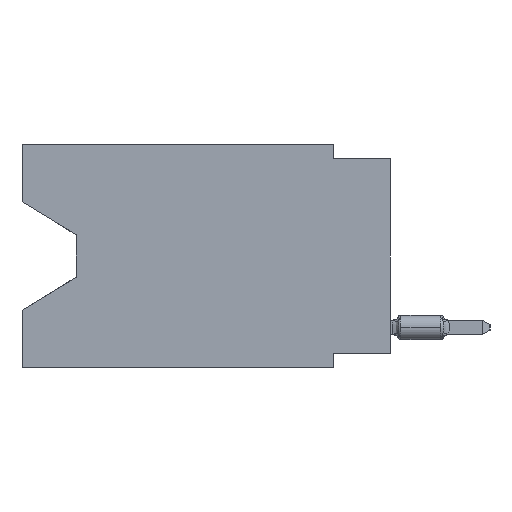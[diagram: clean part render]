
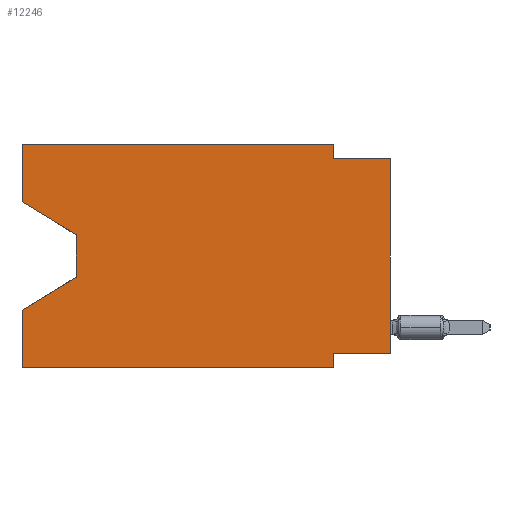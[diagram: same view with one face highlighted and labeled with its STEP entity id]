
A CAD part, left-side view. The second image highlights one B-rep face of the part: STEP entity #12246.
In plain terms, the highlighted planar face has unit normal (-1, 0, 0).
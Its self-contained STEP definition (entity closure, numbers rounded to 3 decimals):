
#37 = LINE ( 'NONE', #5600, #20812 ) ;
#146 = CARTESIAN_POINT ( 'NONE',  ( 0., 13.97, -4.013 ) ) ;
#242 = EDGE_CURVE ( 'NONE', #9040, #10524, #37, .T. ) ;
#517 = VECTOR ( 'NONE', #4023, 1000. ) ;
#622 = ORIENTED_EDGE ( 'NONE', *, *, #14568, .F. ) ;
#646 = EDGE_CURVE ( 'NONE', #13776, #15705, #7178, .T. ) ;
#721 = ORIENTED_EDGE ( 'NONE', *, *, #16237, .T. ) ;
#1942 = CARTESIAN_POINT ( 'NONE',  ( 0., 16.383, 0. ) ) ;
#2270 = CARTESIAN_POINT ( 'NONE',  ( 0., 13.97, -5.893 ) ) ;
#2625 = EDGE_LOOP ( 'NONE', ( #17811, #4729, #721, #22074, #13948, #11797, #7082, #12581, #9591, #7500, #12190, #622 ) ) ;
#2692 = EDGE_CURVE ( 'NONE', #9040, #7118, #13014, .T. ) ;
#3047 = DIRECTION ( 'NONE',  ( 0., -0.855, -0.519 ) ) ;
#3418 = VECTOR ( 'NONE', #3047, 1000. ) ;
#3600 = DIRECTION ( 'NONE',  ( 0., 0., -1. ) ) ;
#4023 = DIRECTION ( 'NONE',  ( 0., -1., 0. ) ) ;
#4031 = CARTESIAN_POINT ( 'NONE',  ( 0., 0., 0. ) ) ;
#4041 = VECTOR ( 'NONE', #5174, 1000. ) ;
#4201 = VECTOR ( 'NONE', #17348, 1000. ) ;
#4598 = DIRECTION ( 'NONE',  ( 1., 0., 0. ) ) ;
#4729 = ORIENTED_EDGE ( 'NONE', *, *, #12365, .T. ) ;
#5174 = DIRECTION ( 'NONE',  ( 0., 0., -1. ) ) ;
#5590 = DIRECTION ( 'NONE',  ( 0., 0., -1. ) ) ;
#5600 = CARTESIAN_POINT ( 'NONE',  ( 0., 0., -9.271 ) ) ;
#5943 = LINE ( 'NONE', #12563, #517 ) ;
#6229 = CARTESIAN_POINT ( 'NONE',  ( 0., 16.383, -2.546 ) ) ;
#6346 = VECTOR ( 'NONE', #9204, 1000. ) ;
#6535 = LINE ( 'NONE', #8246, #18710 ) ;
#6581 = VERTEX_POINT ( 'NONE', #6779 ) ;
#6779 = CARTESIAN_POINT ( 'NONE',  ( 0., 16.383, -2.546 ) ) ;
#6916 = VERTEX_POINT ( 'NONE', #9575 ) ;
#6976 = CARTESIAN_POINT ( 'NONE',  ( 0., 2.54, 0. ) ) ;
#7082 = ORIENTED_EDGE ( 'NONE', *, *, #242, .F. ) ;
#7118 = VERTEX_POINT ( 'NONE', #20900 ) ;
#7178 = LINE ( 'NONE', #1942, #19442 ) ;
#7400 = VECTOR ( 'NONE', #19209, 1000. ) ;
#7429 = CARTESIAN_POINT ( 'NONE',  ( 0., 13.97, -4.013 ) ) ;
#7500 = ORIENTED_EDGE ( 'NONE', *, *, #9701, .F. ) ;
#8246 = CARTESIAN_POINT ( 'NONE',  ( 0., 0., -0.635 ) ) ;
#8387 = LINE ( 'NONE', #6229, #3418 ) ;
#9040 = VERTEX_POINT ( 'NONE', #21508 ) ;
#9204 = DIRECTION ( 'NONE',  ( 0., 0.855, -0.519 ) ) ;
#9448 = EDGE_CURVE ( 'NONE', #10524, #11047, #13818, .T. ) ;
#9575 = CARTESIAN_POINT ( 'NONE',  ( 0., 2.54, -0.635 ) ) ;
#9591 = ORIENTED_EDGE ( 'NONE', *, *, #19391, .F. ) ;
#9643 = AXIS2_PLACEMENT_3D ( 'NONE', #20108, #4598, #11529 ) ;
#9701 = EDGE_CURVE ( 'NONE', #15705, #6916, #14254, .T. ) ;
#9967 = VERTEX_POINT ( 'NONE', #13903 ) ;
#10524 = VERTEX_POINT ( 'NONE', #15392 ) ;
#10589 = VERTEX_POINT ( 'NONE', #7429 ) ;
#10631 = EDGE_CURVE ( 'NONE', #19142, #11047, #5943, .T. ) ;
#10908 = CARTESIAN_POINT ( 'NONE',  ( 0., 16.383, -7.36 ) ) ;
#11047 = VERTEX_POINT ( 'NONE', #15025 ) ;
#11529 = DIRECTION ( 'NONE',  ( 0., 0., -1. ) ) ;
#11647 = DIRECTION ( 'NONE',  ( 0., -1., 0. ) ) ;
#11797 = ORIENTED_EDGE ( 'NONE', *, *, #9448, .F. ) ;
#12190 = ORIENTED_EDGE ( 'NONE', *, *, #646, .F. ) ;
#12246 = ADVANCED_FACE ( 'NONE', ( #21905 ), #18520, .F. ) ;
#12330 = CARTESIAN_POINT ( 'NONE',  ( 0., 16.383, 0. ) ) ;
#12365 = EDGE_CURVE ( 'NONE', #10589, #9967, #15928, .T. ) ;
#12563 = CARTESIAN_POINT ( 'NONE',  ( 0., 16.383, -9.906 ) ) ;
#12581 = ORIENTED_EDGE ( 'NONE', *, *, #2692, .T. ) ;
#12896 = DIRECTION ( 'NONE',  ( 0., 0., 1. ) ) ;
#13014 = LINE ( 'NONE', #4031, #21427 ) ;
#13776 = VERTEX_POINT ( 'NONE', #14787 ) ;
#13818 = LINE ( 'NONE', #15523, #4041 ) ;
#13903 = CARTESIAN_POINT ( 'NONE',  ( 0., 13.97, -5.893 ) ) ;
#13948 = ORIENTED_EDGE ( 'NONE', *, *, #10631, .T. ) ;
#14254 = LINE ( 'NONE', #19456, #21388 ) ;
#14270 = EDGE_CURVE ( 'NONE', #6581, #10589, #8387, .T. ) ;
#14568 = EDGE_CURVE ( 'NONE', #6581, #13776, #19112, .T. ) ;
#14787 = CARTESIAN_POINT ( 'NONE',  ( 0., 16.383, 0. ) ) ;
#15025 = CARTESIAN_POINT ( 'NONE',  ( 0., 2.54, -9.906 ) ) ;
#15392 = CARTESIAN_POINT ( 'NONE',  ( 0., 2.54, -9.271 ) ) ;
#15523 = CARTESIAN_POINT ( 'NONE',  ( 0., 2.54, -9.906 ) ) ;
#15705 = VERTEX_POINT ( 'NONE', #6976 ) ;
#15928 = LINE ( 'NONE', #146, #17259 ) ;
#15938 = DIRECTION ( 'NONE',  ( 0., 1., 0. ) ) ;
#16237 = EDGE_CURVE ( 'NONE', #9967, #20154, #19091, .T. ) ;
#16505 = EDGE_CURVE ( 'NONE', #19142, #20154, #21981, .T. ) ;
#16924 = CARTESIAN_POINT ( 'NONE',  ( 0., 16.383, 0. ) ) ;
#17259 = VECTOR ( 'NONE', #5590, 1000. ) ;
#17348 = DIRECTION ( 'NONE',  ( 0., 0., 1. ) ) ;
#17713 = DIRECTION ( 'NONE',  ( 0., -1., 0. ) ) ;
#17811 = ORIENTED_EDGE ( 'NONE', *, *, #14270, .T. ) ;
#18520 = PLANE ( 'NONE',  #9643 ) ;
#18710 = VECTOR ( 'NONE', #11647, 1000. ) ;
#19091 = LINE ( 'NONE', #2270, #6346 ) ;
#19112 = LINE ( 'NONE', #12330, #7400 ) ;
#19142 = VERTEX_POINT ( 'NONE', #19239 ) ;
#19209 = DIRECTION ( 'NONE',  ( 0., 0., 1. ) ) ;
#19239 = CARTESIAN_POINT ( 'NONE',  ( 0., 16.383, -9.906 ) ) ;
#19391 = EDGE_CURVE ( 'NONE', #6916, #7118, #6535, .T. ) ;
#19442 = VECTOR ( 'NONE', #17713, 1000. ) ;
#19456 = CARTESIAN_POINT ( 'NONE',  ( 0., 2.54, 0. ) ) ;
#20108 = CARTESIAN_POINT ( 'NONE',  ( 0., 16.383, 0. ) ) ;
#20154 = VERTEX_POINT ( 'NONE', #10908 ) ;
#20812 = VECTOR ( 'NONE', #15938, 1000. ) ;
#20900 = CARTESIAN_POINT ( 'NONE',  ( 0., 0., -0.635 ) ) ;
#21388 = VECTOR ( 'NONE', #3600, 1000. ) ;
#21427 = VECTOR ( 'NONE', #12896, 1000. ) ;
#21508 = CARTESIAN_POINT ( 'NONE',  ( 0., 0., -9.271 ) ) ;
#21905 = FACE_OUTER_BOUND ( 'NONE', #2625, .T. ) ;
#21981 = LINE ( 'NONE', #16924, #4201 ) ;
#22074 = ORIENTED_EDGE ( 'NONE', *, *, #16505, .F. ) ;
